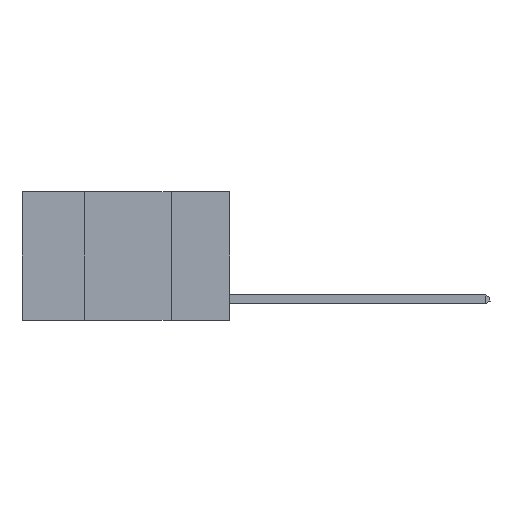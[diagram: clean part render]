
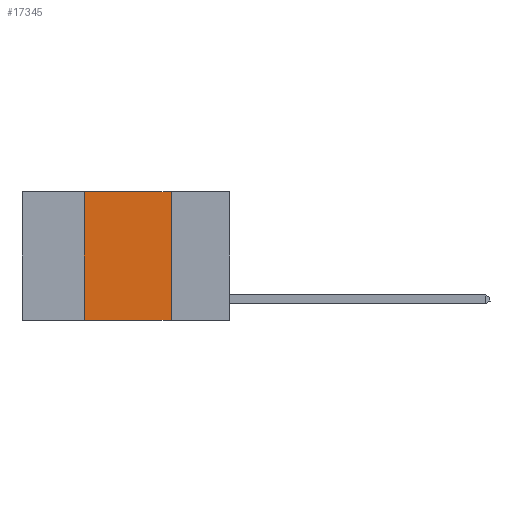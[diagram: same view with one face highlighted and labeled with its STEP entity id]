
A CAD part, left-side view. The second image highlights one B-rep face of the part: STEP entity #17345.
In plain terms, the highlighted planar face has unit normal (-1, 0, 0).
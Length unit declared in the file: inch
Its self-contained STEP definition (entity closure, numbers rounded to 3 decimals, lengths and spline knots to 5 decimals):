
#292 = CARTESIAN_POINT ( 'NONE',  ( 0., 0.42, 0. ) ) ;
#746 = VECTOR ( 'NONE', #4902, 39.37008 ) ;
#1260 = AXIS2_PLACEMENT_3D ( 'NONE', #16393, #3646, #13575 ) ;
#2314 = LINE ( 'NONE', #8568, #16995 ) ;
#2960 = DIRECTION ( 'NONE',  ( 0., -1., 0. ) ) ;
#3646 = DIRECTION ( 'NONE',  ( 1., 0., 0. ) ) ;
#4041 = ORIENTED_EDGE ( 'NONE', *, *, #15301, .F. ) ;
#4344 = DIRECTION ( 'NONE',  ( 0., -1., 0. ) ) ;
#4869 = CARTESIAN_POINT ( 'NONE',  ( 0., 0.17, 0. ) ) ;
#4902 = DIRECTION ( 'NONE',  ( 0., 0., 1. ) ) ;
#5015 = VECTOR ( 'NONE', #2960, 39.37008 ) ;
#5026 = CARTESIAN_POINT ( 'NONE',  ( 0., 0.42, -0.37 ) ) ;
#5258 = VERTEX_POINT ( 'NONE', #292 ) ;
#6352 = CARTESIAN_POINT ( 'NONE',  ( 0., 0.42, 0. ) ) ;
#6670 = EDGE_CURVE ( 'NONE', #10544, #18289, #16341, .T. ) ;
#7199 = CARTESIAN_POINT ( 'NONE',  ( 0., 0.6, -0.37 ) ) ;
#8166 = ORIENTED_EDGE ( 'NONE', *, *, #10468, .F. ) ;
#8568 = CARTESIAN_POINT ( 'NONE',  ( 0., 0.6, 0. ) ) ;
#9724 = ORIENTED_EDGE ( 'NONE', *, *, #16660, .F. ) ;
#10468 = EDGE_CURVE ( 'NONE', #10544, #5258, #12163, .T. ) ;
#10544 = VERTEX_POINT ( 'NONE', #5026 ) ;
#10586 = DIRECTION ( 'NONE',  ( 0., 0., -1. ) ) ;
#11404 = VECTOR ( 'NONE', #10586, 39.37008 ) ;
#11465 = ORIENTED_EDGE ( 'NONE', *, *, #6670, .T. ) ;
#11913 = VERTEX_POINT ( 'NONE', #14470 ) ;
#12112 = PLANE ( 'NONE',  #1260 ) ;
#12163 = LINE ( 'NONE', #6352, #746 ) ;
#13575 = DIRECTION ( 'NONE',  ( 0., 0., -1. ) ) ;
#14470 = CARTESIAN_POINT ( 'NONE',  ( 0., 0.17, 0. ) ) ;
#15164 = LINE ( 'NONE', #4869, #11404 ) ;
#15301 = EDGE_CURVE ( 'NONE', #5258, #11913, #2314, .T. ) ;
#16341 = LINE ( 'NONE', #7199, #5015 ) ;
#16393 = CARTESIAN_POINT ( 'NONE',  ( 0., 0.6, 0. ) ) ;
#16485 = EDGE_LOOP ( 'NONE', ( #9724, #4041, #8166, #11465 ) ) ;
#16660 = EDGE_CURVE ( 'NONE', #11913, #18289, #15164, .T. ) ;
#16995 = VECTOR ( 'NONE', #4344, 39.37008 ) ;
#17345 = ADVANCED_FACE ( 'NONE', ( #17811 ), #12112, .F. ) ;
#17811 = FACE_OUTER_BOUND ( 'NONE', #16485, .T. ) ;
#17947 = CARTESIAN_POINT ( 'NONE',  ( 0., 0.17, -0.37 ) ) ;
#18289 = VERTEX_POINT ( 'NONE', #17947 ) ;
